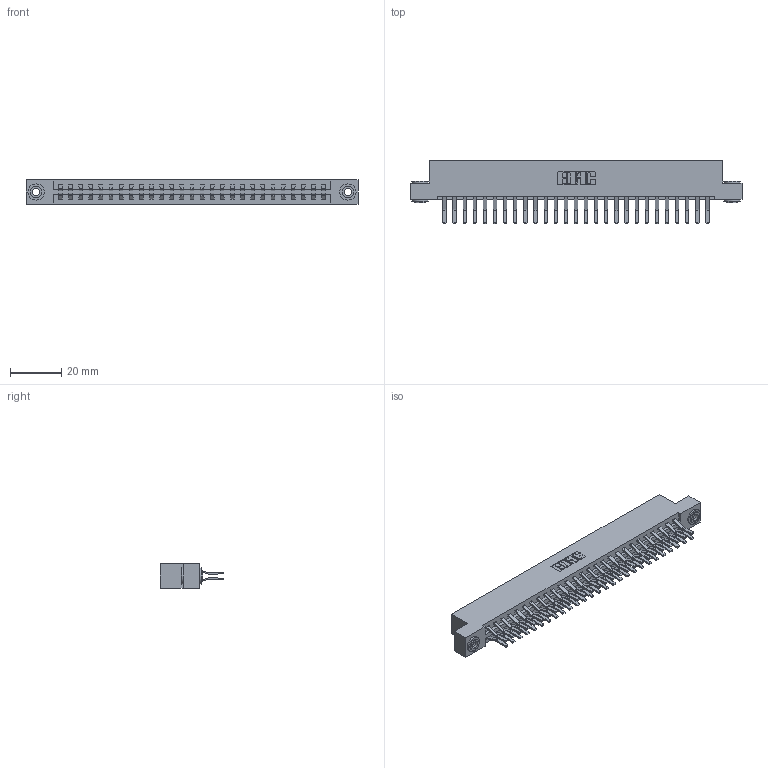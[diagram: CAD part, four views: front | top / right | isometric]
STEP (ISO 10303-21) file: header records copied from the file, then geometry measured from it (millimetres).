
FILE_DESCRIPTION (( 'STEP AP203' ), '1' );
FILE_NAME ('387-054-560-203.STEP', '2019-10-19T06:00:19', ( '' ), ( '' ), 'SwSTEP 2.0', 'SolidWorks 2016', '' );
FILE_SCHEMA (( 'CONFIG_CONTROL_DESIGN' ));
Length unit declared in the file: inch
Products named in the file (4): 387-054-560-203; 345-292-001_560 Tail; 337 Part_Flush Mounting Lugs - 0.156 Dia-TH; 345-250-002_345-250-002-102
Assembly tree (57 placements, depth 2):
  387-054-560-203
    337 Part_Flush Mounting Lugs - 0.156 Dia-TH
    345-292-001_560 Tail  x54
    345-250-002_345-250-002-102  x2
Bounding box: 130 x 24.78 x 9.4 mm (x, y, z)
Volume: 13873.8 mm3; surface area: 16787.5 mm2
Topology: 57 solids, 57 shells, 3176 faces, 9405 edges, 6194 vertices
Faces by surface type: plane 2132, cylinder 1036, cone 8
Entity records: 23612 total; most frequent: CARTESIAN_POINT 3965, ORIENTED_EDGE 3894, DIRECTION 3437, EDGE_CURVE 1947, LINE 1791, VECTOR 1791, VERTEX_POINT 1294, AXIS2_PLACEMENT_3D 823
